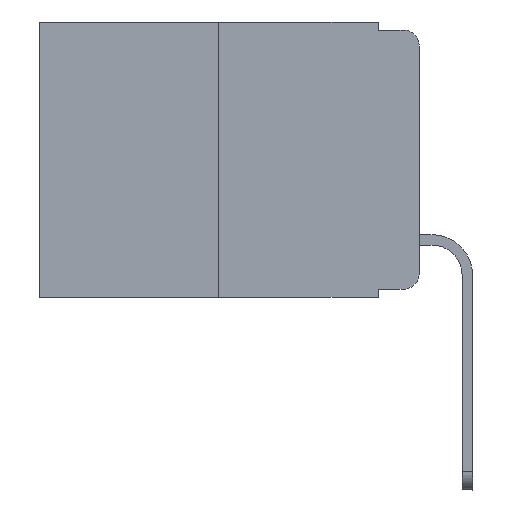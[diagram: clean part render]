
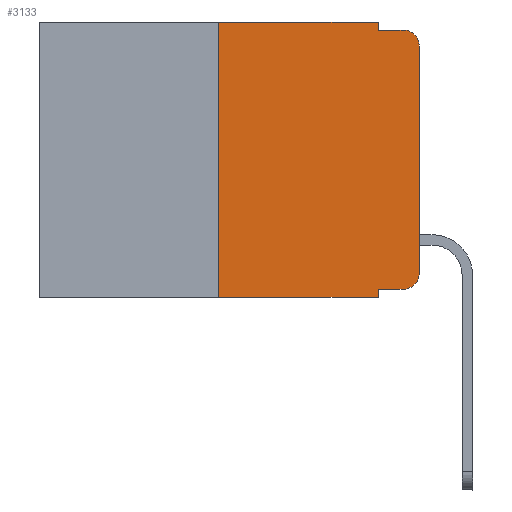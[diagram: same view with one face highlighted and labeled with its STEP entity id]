
A CAD part, left-side view. The second image highlights one B-rep face of the part: STEP entity #3133.
In plain terms, the highlighted planar face has unit normal (-1, 0, 0).
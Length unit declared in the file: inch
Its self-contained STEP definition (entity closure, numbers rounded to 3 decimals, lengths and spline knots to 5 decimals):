
#263 = VERTEX_POINT ( 'NONE', #9185 ) ;
#772 = LINE ( 'NONE', #4881, #11755 ) ;
#800 = VERTEX_POINT ( 'NONE', #1968 ) ;
#832 = EDGE_CURVE ( 'NONE', #263, #800, #9394, .T. ) ;
#936 = EDGE_CURVE ( 'NONE', #11811, #11192, #1173, .T. ) ;
#1082 = LINE ( 'NONE', #10499, #10067 ) ;
#1123 = CARTESIAN_POINT ( 'NONE',  ( 0., 0.473, 0. ) ) ;
#1164 = LINE ( 'NONE', #1288, #8574 ) ;
#1173 = CIRCLE ( 'NONE', #8750, 0.02 ) ;
#1215 = ORIENTED_EDGE ( 'NONE', *, *, #2329, .F. ) ;
#1288 = CARTESIAN_POINT ( 'NONE',  ( 0., 0.473, 0. ) ) ;
#1422 = ORIENTED_EDGE ( 'NONE', *, *, #9524, .F. ) ;
#1843 = DIRECTION ( 'NONE',  ( 0., 0., -1. ) ) ;
#1968 = CARTESIAN_POINT ( 'NONE',  ( 0., 0.02, -0.01 ) ) ;
#2000 = DIRECTION ( 'NONE',  ( 1., 0., 0. ) ) ;
#2183 = CARTESIAN_POINT ( 'NONE',  ( 0., 0.051, 0. ) ) ;
#2199 = DIRECTION ( 'NONE',  ( 0., -1., 0. ) ) ;
#2284 = CARTESIAN_POINT ( 'NONE',  ( 0., 0.02, -0.313 ) ) ;
#2329 = EDGE_CURVE ( 'NONE', #8587, #10562, #1164, .T. ) ;
#2412 = ORIENTED_EDGE ( 'NONE', *, *, #8927, .T. ) ;
#2708 = DIRECTION ( 'NONE',  ( -1., 0., 0. ) ) ;
#2836 = CARTESIAN_POINT ( 'NONE',  ( 0., 0.02, -0.03 ) ) ;
#2919 = VECTOR ( 'NONE', #8941, 39.37008 ) ;
#3065 = DIRECTION ( 'NONE',  ( 0., 0., -1. ) ) ;
#3133 = ADVANCED_FACE ( 'NONE', ( #9392 ), #8369, .F. ) ;
#3648 = CARTESIAN_POINT ( 'NONE',  ( 0., 0.051, -0.343 ) ) ;
#3870 = ORIENTED_EDGE ( 'NONE', *, *, #832, .T. ) ;
#4282 = CARTESIAN_POINT ( 'NONE',  ( 0., 0.051, 0. ) ) ;
#4774 = VERTEX_POINT ( 'NONE', #3648 ) ;
#4786 = ORIENTED_EDGE ( 'NONE', *, *, #12998, .T. ) ;
#4881 = CARTESIAN_POINT ( 'NONE',  ( 0., 0.25, 0. ) ) ;
#5050 = AXIS2_PLACEMENT_3D ( 'NONE', #2836, #2708, #1843 ) ;
#5137 = DIRECTION ( 'NONE',  ( -1., 0., 0. ) ) ;
#5278 = VERTEX_POINT ( 'NONE', #7722 ) ;
#5281 = EDGE_LOOP ( 'NONE', ( #2412, #3870, #9362, #6243, #1215, #1422, #4786, #10777, #8754, #7271 ) ) ;
#5339 = DIRECTION ( 'NONE',  ( 0., 0., -1. ) ) ;
#5458 = EDGE_CURVE ( 'NONE', #6977, #11811, #12500, .T. ) ;
#5737 = CARTESIAN_POINT ( 'NONE',  ( 0., 0.051, -0.01 ) ) ;
#6243 = ORIENTED_EDGE ( 'NONE', *, *, #7185, .F. ) ;
#6257 = LINE ( 'NONE', #4282, #12547 ) ;
#6279 = CARTESIAN_POINT ( 'NONE',  ( 0., 0., -0.313 ) ) ;
#6344 = VECTOR ( 'NONE', #10239, 39.37008 ) ;
#6409 = AXIS2_PLACEMENT_3D ( 'NONE', #1123, #2000, #3065 ) ;
#6416 = LINE ( 'NONE', #10559, #7417 ) ;
#6977 = VERTEX_POINT ( 'NONE', #8113 ) ;
#7185 = EDGE_CURVE ( 'NONE', #10562, #10374, #6257, .T. ) ;
#7260 = DIRECTION ( 'NONE',  ( 0., -1., 0. ) ) ;
#7271 = ORIENTED_EDGE ( 'NONE', *, *, #936, .T. ) ;
#7417 = VECTOR ( 'NONE', #10413, 39.37008 ) ;
#7722 = CARTESIAN_POINT ( 'NONE',  ( 0., 0.25, -0.343 ) ) ;
#8113 = CARTESIAN_POINT ( 'NONE',  ( 0., 0.051, -0.333 ) ) ;
#8369 = PLANE ( 'NONE',  #6409 ) ;
#8449 = CARTESIAN_POINT ( 'NONE',  ( 0., 0.051, -0.333 ) ) ;
#8574 = VECTOR ( 'NONE', #7260, 39.37008 ) ;
#8587 = VERTEX_POINT ( 'NONE', #12600 ) ;
#8750 = AXIS2_PLACEMENT_3D ( 'NONE', #2284, #5137, #5339 ) ;
#8754 = ORIENTED_EDGE ( 'NONE', *, *, #5458, .T. ) ;
#8875 = LINE ( 'NONE', #5737, #2919 ) ;
#8927 = EDGE_CURVE ( 'NONE', #11192, #263, #6416, .T. ) ;
#8941 = DIRECTION ( 'NONE',  ( 0., -1., 0. ) ) ;
#9185 = CARTESIAN_POINT ( 'NONE',  ( 0., 0., -0.03 ) ) ;
#9362 = ORIENTED_EDGE ( 'NONE', *, *, #13311, .F. ) ;
#9392 = FACE_OUTER_BOUND ( 'NONE', #5281, .T. ) ;
#9394 = CIRCLE ( 'NONE', #5050, 0.02 ) ;
#9524 = EDGE_CURVE ( 'NONE', #5278, #8587, #772, .T. ) ;
#9694 = EDGE_CURVE ( 'NONE', #6977, #4774, #11195, .T. ) ;
#10067 = VECTOR ( 'NONE', #11445, 39.37008 ) ;
#10142 = VECTOR ( 'NONE', #2199, 39.37008 ) ;
#10168 = CARTESIAN_POINT ( 'NONE',  ( 0., 0.051, 0. ) ) ;
#10239 = DIRECTION ( 'NONE',  ( 0., 0., -1. ) ) ;
#10374 = VERTEX_POINT ( 'NONE', #13102 ) ;
#10402 = DIRECTION ( 'NONE',  ( 0., 0., -1. ) ) ;
#10413 = DIRECTION ( 'NONE',  ( 0., 0., 1. ) ) ;
#10499 = CARTESIAN_POINT ( 'NONE',  ( 0., 0.473, -0.343 ) ) ;
#10559 = CARTESIAN_POINT ( 'NONE',  ( 0., 0., 0. ) ) ;
#10562 = VERTEX_POINT ( 'NONE', #2183 ) ;
#10777 = ORIENTED_EDGE ( 'NONE', *, *, #9694, .F. ) ;
#11192 = VERTEX_POINT ( 'NONE', #6279 ) ;
#11195 = LINE ( 'NONE', #10168, #6344 ) ;
#11445 = DIRECTION ( 'NONE',  ( 0., -1., 0. ) ) ;
#11561 = CARTESIAN_POINT ( 'NONE',  ( 0., 0.02, -0.333 ) ) ;
#11755 = VECTOR ( 'NONE', #12995, 39.37008 ) ;
#11811 = VERTEX_POINT ( 'NONE', #11561 ) ;
#12500 = LINE ( 'NONE', #8449, #10142 ) ;
#12547 = VECTOR ( 'NONE', #10402, 39.37008 ) ;
#12600 = CARTESIAN_POINT ( 'NONE',  ( 0., 0.25, 0. ) ) ;
#12995 = DIRECTION ( 'NONE',  ( 0., 0., 1. ) ) ;
#12998 = EDGE_CURVE ( 'NONE', #5278, #4774, #1082, .T. ) ;
#13102 = CARTESIAN_POINT ( 'NONE',  ( 0., 0.051, -0.01 ) ) ;
#13311 = EDGE_CURVE ( 'NONE', #10374, #800, #8875, .T. ) ;
